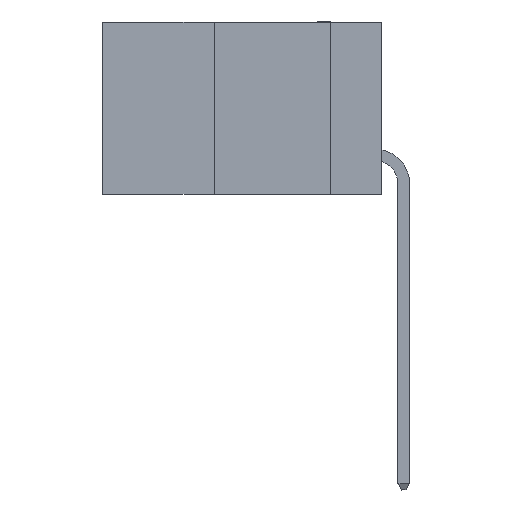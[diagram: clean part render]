
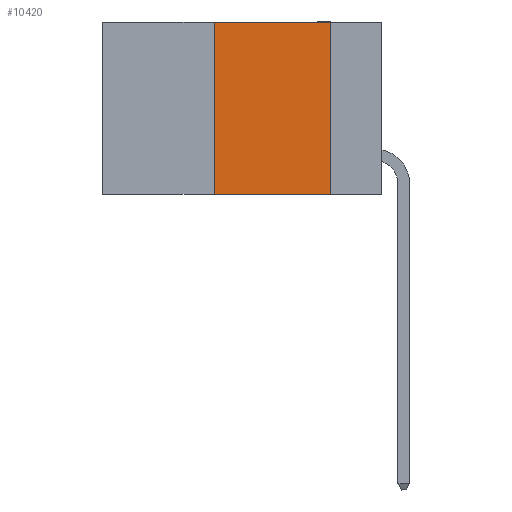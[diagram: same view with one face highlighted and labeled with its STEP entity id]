
A CAD part, left-side view. The second image highlights one B-rep face of the part: STEP entity #10420.
In plain terms, the highlighted planar face has unit normal (-1, 0, 0).
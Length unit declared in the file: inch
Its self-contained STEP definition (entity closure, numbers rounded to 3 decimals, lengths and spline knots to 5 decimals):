
#160 = PLANE ( 'NONE',  #16775 ) ;
#682 = VECTOR ( 'NONE', #11052, 39.37008 ) ;
#1132 = VERTEX_POINT ( 'NONE', #16792 ) ;
#1489 = CARTESIAN_POINT ( 'NONE',  ( 0., 0.36, -0.37 ) ) ;
#2035 = LINE ( 'NONE', #12133, #7079 ) ;
#2362 = CARTESIAN_POINT ( 'NONE',  ( 0., 0.11, 0. ) ) ;
#2566 = VECTOR ( 'NONE', #6851, 39.37008 ) ;
#3920 = VERTEX_POINT ( 'NONE', #2362 ) ;
#4259 = VERTEX_POINT ( 'NONE', #11164 ) ;
#5614 = DIRECTION ( 'NONE',  ( 1., 0., 0. ) ) ;
#6278 = LINE ( 'NONE', #10950, #2566 ) ;
#6851 = DIRECTION ( 'NONE',  ( 0., 0., 1. ) ) ;
#6936 = DIRECTION ( 'NONE',  ( 0., -1., 0. ) ) ;
#7019 = EDGE_LOOP ( 'NONE', ( #15711, #9021, #16020, #11049 ) ) ;
#7079 = VECTOR ( 'NONE', #9305, 39.37008 ) ;
#9021 = ORIENTED_EDGE ( 'NONE', *, *, #18081, .F. ) ;
#9305 = DIRECTION ( 'NONE',  ( 0., 0., -1. ) ) ;
#9674 = EDGE_CURVE ( 'NONE', #16325, #1132, #6278, .T. ) ;
#9699 = CARTESIAN_POINT ( 'NONE',  ( 0., 0.6, -0.37 ) ) ;
#10346 = LINE ( 'NONE', #9699, #17595 ) ;
#10420 = ADVANCED_FACE ( 'NONE', ( #17044 ), #160, .F. ) ;
#10744 = LINE ( 'NONE', #11118, #682 ) ;
#10950 = CARTESIAN_POINT ( 'NONE',  ( 0., 0.36, 0. ) ) ;
#11049 = ORIENTED_EDGE ( 'NONE', *, *, #12775, .T. ) ;
#11052 = DIRECTION ( 'NONE',  ( 0., -1., 0. ) ) ;
#11118 = CARTESIAN_POINT ( 'NONE',  ( 0., 0.6, 0. ) ) ;
#11164 = CARTESIAN_POINT ( 'NONE',  ( 0., 0.11, -0.37 ) ) ;
#12133 = CARTESIAN_POINT ( 'NONE',  ( 0., 0.11, 0. ) ) ;
#12775 = EDGE_CURVE ( 'NONE', #16325, #4259, #10346, .T. ) ;
#12836 = DIRECTION ( 'NONE',  ( 0., 0., -1. ) ) ;
#15491 = CARTESIAN_POINT ( 'NONE',  ( 0., 0.6, 0. ) ) ;
#15711 = ORIENTED_EDGE ( 'NONE', *, *, #16713, .F. ) ;
#16020 = ORIENTED_EDGE ( 'NONE', *, *, #9674, .F. ) ;
#16325 = VERTEX_POINT ( 'NONE', #1489 ) ;
#16713 = EDGE_CURVE ( 'NONE', #3920, #4259, #2035, .T. ) ;
#16775 = AXIS2_PLACEMENT_3D ( 'NONE', #15491, #5614, #12836 ) ;
#16792 = CARTESIAN_POINT ( 'NONE',  ( 0., 0.36, 0. ) ) ;
#17044 = FACE_OUTER_BOUND ( 'NONE', #7019, .T. ) ;
#17595 = VECTOR ( 'NONE', #6936, 39.37008 ) ;
#18081 = EDGE_CURVE ( 'NONE', #1132, #3920, #10744, .T. ) ;
